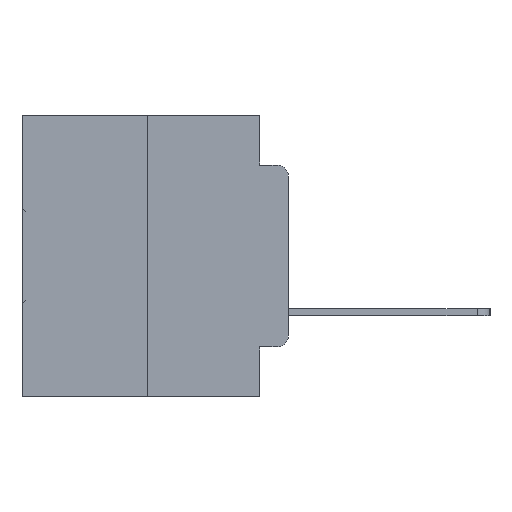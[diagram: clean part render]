
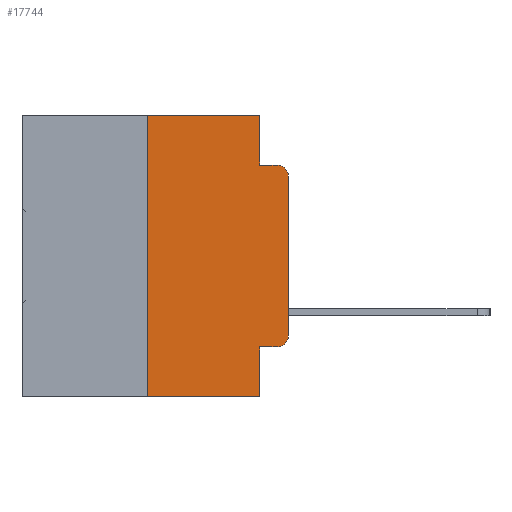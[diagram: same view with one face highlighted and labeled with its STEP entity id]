
A CAD part, left-side view. The second image highlights one B-rep face of the part: STEP entity #17744.
In plain terms, the highlighted planar face has unit normal (-1, 0, 0).
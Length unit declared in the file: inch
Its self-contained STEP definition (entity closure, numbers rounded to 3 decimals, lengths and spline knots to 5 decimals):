
#2133 = VERTEX_POINT ( 'NONE', #23520 ) ;
#2227 = EDGE_CURVE ( 'NONE', #15822, #26527, #28147, .T. ) ;
#2326 = LINE ( 'NONE', #17778, #15762 ) ;
#2396 = CARTESIAN_POINT ( 'NONE',  ( 0., 0.473, 0. ) ) ;
#2556 = CARTESIAN_POINT ( 'NONE',  ( 0., 0.02, -0.3915 ) ) ;
#2658 = DIRECTION ( 'NONE',  ( 0., -1., 0. ) ) ;
#2809 = DIRECTION ( 'NONE',  ( 0., 0., -1. ) ) ;
#2923 = VERTEX_POINT ( 'NONE', #17925 ) ;
#3572 = VERTEX_POINT ( 'NONE', #28154 ) ;
#3848 = CARTESIAN_POINT ( 'NONE',  ( 0., 0.473, -0.5 ) ) ;
#4213 = CIRCLE ( 'NONE', #10782, 0.02 ) ;
#5108 = DIRECTION ( 'NONE',  ( 0., 0., -1. ) ) ;
#5394 = LINE ( 'NONE', #15637, #24647 ) ;
#6692 = DIRECTION ( 'NONE',  ( -1., 0., 0. ) ) ;
#7519 = DIRECTION ( 'NONE',  ( 1., 0., 0. ) ) ;
#7625 = CARTESIAN_POINT ( 'NONE',  ( 0., 0.051, -0.0885 ) ) ;
#7937 = VECTOR ( 'NONE', #18053, 39.37008 ) ;
#8151 = ORIENTED_EDGE ( 'NONE', *, *, #23929, .T. ) ;
#8184 = VECTOR ( 'NONE', #29880, 39.37008 ) ;
#8824 = CARTESIAN_POINT ( 'NONE',  ( 0., 0.02, -0.0885 ) ) ;
#8953 = VERTEX_POINT ( 'NONE', #31572 ) ;
#9978 = EDGE_CURVE ( 'NONE', #15822, #2133, #5394, .T. ) ;
#10198 = AXIS2_PLACEMENT_3D ( 'NONE', #2556, #20221, #5108 ) ;
#10249 = EDGE_CURVE ( 'NONE', #3572, #20068, #4213, .T. ) ;
#10782 = AXIS2_PLACEMENT_3D ( 'NONE', #21729, #6692, #24211 ) ;
#11321 = DIRECTION ( 'NONE',  ( 0., 0., 1. ) ) ;
#12055 = EDGE_CURVE ( 'NONE', #2923, #26527, #16716, .T. ) ;
#12431 = CIRCLE ( 'NONE', #10198, 0.02 ) ;
#12915 = ORIENTED_EDGE ( 'NONE', *, *, #16751, .F. ) ;
#13009 = CARTESIAN_POINT ( 'NONE',  ( 0., 0.051, 0. ) ) ;
#13117 = VERTEX_POINT ( 'NONE', #7625 ) ;
#13234 = CARTESIAN_POINT ( 'NONE',  ( 0., 0.25, -0.5 ) ) ;
#13497 = VECTOR ( 'NONE', #11321, 39.37008 ) ;
#14109 = ORIENTED_EDGE ( 'NONE', *, *, #12055, .F. ) ;
#14490 = ORIENTED_EDGE ( 'NONE', *, *, #24296, .F. ) ;
#14648 = LINE ( 'NONE', #15542, #7937 ) ;
#15251 = EDGE_LOOP ( 'NONE', ( #8151, #21502, #12915, #19604, #14490, #27758, #16843, #14109, #27378, #22293 ) ) ;
#15365 = EDGE_CURVE ( 'NONE', #2923, #16608, #24017, .T. ) ;
#15542 = CARTESIAN_POINT ( 'NONE',  ( 0., 0.051, -0.0885 ) ) ;
#15637 = CARTESIAN_POINT ( 'NONE',  ( 0., 0.25, 0. ) ) ;
#15762 = VECTOR ( 'NONE', #2658, 39.37008 ) ;
#15822 = VERTEX_POINT ( 'NONE', #13234 ) ;
#15908 = VECTOR ( 'NONE', #25946, 39.37008 ) ;
#16422 = CARTESIAN_POINT ( 'NONE',  ( 0., 0.051, -0.4115 ) ) ;
#16608 = VERTEX_POINT ( 'NONE', #24912 ) ;
#16716 = LINE ( 'NONE', #23413, #15908 ) ;
#16751 = EDGE_CURVE ( 'NONE', #13117, #20068, #14648, .T. ) ;
#16843 = ORIENTED_EDGE ( 'NONE', *, *, #2227, .T. ) ;
#16922 = VECTOR ( 'NONE', #2809, 39.37008 ) ;
#17744 = ADVANCED_FACE ( 'NONE', ( #32085 ), #29926, .F. ) ;
#17778 = CARTESIAN_POINT ( 'NONE',  ( 0., 0.473, 0. ) ) ;
#17925 = CARTESIAN_POINT ( 'NONE',  ( 0., 0.051, -0.4115 ) ) ;
#18053 = DIRECTION ( 'NONE',  ( 0., -1., 0. ) ) ;
#18153 = DIRECTION ( 'NONE',  ( 0., 0., 1. ) ) ;
#18731 = VERTEX_POINT ( 'NONE', #28795 ) ;
#18977 = DIRECTION ( 'NONE',  ( 0., -1., 0. ) ) ;
#19604 = ORIENTED_EDGE ( 'NONE', *, *, #31936, .F. ) ;
#20068 = VERTEX_POINT ( 'NONE', #8824 ) ;
#20221 = DIRECTION ( 'NONE',  ( -1., 0., 0. ) ) ;
#20235 = CARTESIAN_POINT ( 'NONE',  ( 0., 0.051, -0.5 ) ) ;
#21502 = ORIENTED_EDGE ( 'NONE', *, *, #10249, .T. ) ;
#21729 = CARTESIAN_POINT ( 'NONE',  ( 0., 0.02, -0.1085 ) ) ;
#22293 = ORIENTED_EDGE ( 'NONE', *, *, #22414, .T. ) ;
#22414 = EDGE_CURVE ( 'NONE', #16608, #18731, #12431, .T. ) ;
#23219 = VECTOR ( 'NONE', #18977, 39.37008 ) ;
#23413 = CARTESIAN_POINT ( 'NONE',  ( 0., 0.051, 0. ) ) ;
#23520 = CARTESIAN_POINT ( 'NONE',  ( 0., 0.25, 0. ) ) ;
#23929 = EDGE_CURVE ( 'NONE', #18731, #3572, #24885, .T. ) ;
#24017 = LINE ( 'NONE', #16422, #23219 ) ;
#24211 = DIRECTION ( 'NONE',  ( 0., 0., -1. ) ) ;
#24296 = EDGE_CURVE ( 'NONE', #2133, #8953, #2326, .T. ) ;
#24647 = VECTOR ( 'NONE', #18153, 39.37008 ) ;
#24885 = LINE ( 'NONE', #31143, #13497 ) ;
#24912 = CARTESIAN_POINT ( 'NONE',  ( 0., 0.02, -0.4115 ) ) ;
#25034 = DIRECTION ( 'NONE',  ( 0., 0., -1. ) ) ;
#25946 = DIRECTION ( 'NONE',  ( 0., 0., -1. ) ) ;
#26527 = VERTEX_POINT ( 'NONE', #20235 ) ;
#27378 = ORIENTED_EDGE ( 'NONE', *, *, #15365, .T. ) ;
#27758 = ORIENTED_EDGE ( 'NONE', *, *, #9978, .F. ) ;
#27905 = AXIS2_PLACEMENT_3D ( 'NONE', #2396, #7519, #25034 ) ;
#28147 = LINE ( 'NONE', #3848, #8184 ) ;
#28154 = CARTESIAN_POINT ( 'NONE',  ( 0., 0., -0.1085 ) ) ;
#28795 = CARTESIAN_POINT ( 'NONE',  ( 0., 0., -0.3915 ) ) ;
#29880 = DIRECTION ( 'NONE',  ( 0., -1., 0. ) ) ;
#29926 = PLANE ( 'NONE',  #27905 ) ;
#30140 = LINE ( 'NONE', #13009, #16922 ) ;
#31143 = CARTESIAN_POINT ( 'NONE',  ( 0., 0., 0. ) ) ;
#31572 = CARTESIAN_POINT ( 'NONE',  ( 0., 0.051, 0. ) ) ;
#31936 = EDGE_CURVE ( 'NONE', #8953, #13117, #30140, .T. ) ;
#32085 = FACE_OUTER_BOUND ( 'NONE', #15251, .T. ) ;
